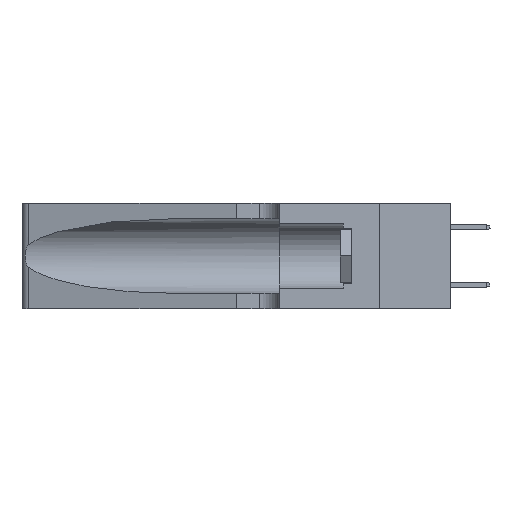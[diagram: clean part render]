
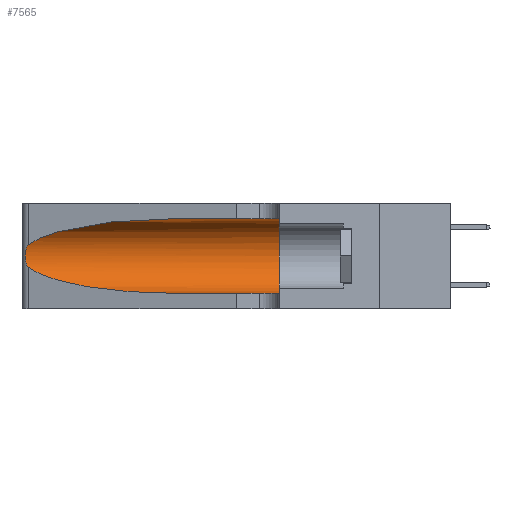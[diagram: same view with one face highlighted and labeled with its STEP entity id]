
A CAD part, left-side view. The second image highlights one B-rep face of the part: STEP entity #7565.
In plain terms, the highlighted cylindrical face has radius 3.308 mm (diameter 6.617 mm), a partial arc.
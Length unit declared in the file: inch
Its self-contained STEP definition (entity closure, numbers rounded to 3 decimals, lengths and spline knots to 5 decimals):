
#405 =( BOUNDED_CURVE ( )  B_SPLINE_CURVE ( 3, ( #37373, #41398, #25965, #8389 ),
 .UNSPECIFIED., .F., .T. ) 
 B_SPLINE_CURVE_WITH_KNOTS ( ( 4, 4 ),
 ( 1.5708, 2.84003 ),
 .UNSPECIFIED. ) 
 CURVE ( )  GEOMETRIC_REPRESENTATION_ITEM ( )  RATIONAL_B_SPLINE_CURVE ( ( 1., 0.87, 0.87, 1. ) ) 
 REPRESENTATION_ITEM ( '' )  );
#456 = CARTESIAN_POINT ( 'NONE',  ( 0.1305, 1.61858, 0.185 ) ) ;
#863 = DIRECTION ( 'NONE',  ( 0., -1., 0. ) ) ;
#1605 = CARTESIAN_POINT ( 'NONE',  ( 0.1305, 0.72297, 0.05475 ) ) ;
#2147 = CIRCLE ( 'NONE', #30199, 0.13025 ) ;
#2253 = CARTESIAN_POINT ( 'NONE',  ( 0.1305, 0.72297, 0.31525 ) ) ;
#2636 = EDGE_CURVE ( 'NONE', #8098, #27997, #2147, .T. ) ;
#3401 = CARTESIAN_POINT ( 'NONE',  ( 0.25789, 1.23486, 0.15765 ) ) ;
#3547 = EDGE_CURVE ( 'NONE', #12469, #27997, #24114, .T. ) ;
#4319 = EDGE_CURVE ( 'NONE', #40891, #12469, #14695, .T. ) ;
#4359 = CARTESIAN_POINT ( 'NONE',  ( 0.1305, 0.72297, 0.05475 ) ) ;
#4666 = LINE ( 'NONE', #18944, #4893 ) ;
#4893 = VECTOR ( 'NONE', #863, 39.37008 ) ;
#6642 = CARTESIAN_POINT ( 'NONE',  ( 0.1305, 0.35, 0.185 ) ) ;
#6947 = CARTESIAN_POINT ( 'NONE',  ( 0.26017, 1.23833, 0.17102 ) ) ;
#7431 = CARTESIAN_POINT ( 'NONE',  ( 0.26018, 1.23835, 0.19895 ) ) ;
#7565 = ADVANCED_FACE ( 'NONE', ( #22329 ), #33008, .F. ) ;
#8098 = VERTEX_POINT ( 'NONE', #11119 ) ;
#8389 = CARTESIAN_POINT ( 'NONE',  ( 0.25487, 1.22718, 0.22369 ) ) ;
#8571 = EDGE_LOOP ( 'NONE', ( #9879, #26465, #32762, #14339, #31455, #34783 ) ) ;
#9879 = ORIENTED_EDGE ( 'NONE', *, *, #27897, .T. ) ;
#10057 = VERTEX_POINT ( 'NONE', #12713 ) ;
#11119 = CARTESIAN_POINT ( 'NONE',  ( 0.1305, 0.35, 0.31525 ) ) ;
#12469 = VERTEX_POINT ( 'NONE', #4359 ) ;
#12713 = CARTESIAN_POINT ( 'NONE',  ( 0.25487, 1.22718, 0.22369 ) ) ;
#13401 = CARTESIAN_POINT ( 'NONE',  ( 0.25487, 1.22718, 0.22369 ) ) ;
#14079 = EDGE_CURVE ( 'NONE', #10057, #40891, #15015, .T. ) ;
#14339 = ORIENTED_EDGE ( 'NONE', *, *, #3547, .T. ) ;
#14544 = CARTESIAN_POINT ( 'NONE',  ( 0.25555, 1.22993, 0.14849 ) ) ;
#14695 =( BOUNDED_CURVE ( )  B_SPLINE_CURVE ( 3, ( #37728, #19687, #34153, #1605 ),
 .UNSPECIFIED., .F., .F. ) 
 B_SPLINE_CURVE_WITH_KNOTS ( ( 4, 4 ),
 ( 3.44316, 4.71239 ),
 .UNSPECIFIED. ) 
 CURVE ( )  GEOMETRIC_REPRESENTATION_ITEM ( )  RATIONAL_B_SPLINE_CURVE ( ( 1., 0.87, 0.87, 1. ) ) 
 REPRESENTATION_ITEM ( '' )  );
#15015 = B_SPLINE_CURVE_WITH_KNOTS ( 'NONE', 3,
 ( #13401, #27882, #42360, #38810, #20784, #7431, #21231, #43064, #6947, #24557, #3401, #36400, #14544, #18153 ),
 .UNSPECIFIED., .F., .F.,
 ( 4, 2, 2, 2, 2, 2, 4 ),
 ( 0., 0.00027, 0.00053, 0.00107, 0.0016, 0.00187, 0.00214 ),
 .UNSPECIFIED. ) ;
#16765 = CARTESIAN_POINT ( 'NONE',  ( 0.1305, 1.61858, 0.05475 ) ) ;
#18153 = CARTESIAN_POINT ( 'NONE',  ( 0.25487, 1.22718, 0.14631 ) ) ;
#18765 = DIRECTION ( 'NONE',  ( 0., 0., -1. ) ) ;
#18944 = CARTESIAN_POINT ( 'NONE',  ( 0.1305, 1.61858, 0.31525 ) ) ;
#19687 = CARTESIAN_POINT ( 'NONE',  ( 0.2373, 1.15595, 0.08982 ) ) ;
#20686 = DIRECTION ( 'NONE',  ( 0., 1., 0. ) ) ;
#20784 = CARTESIAN_POINT ( 'NONE',  ( 0.25854, 1.2359, 0.20912 ) ) ;
#21231 = CARTESIAN_POINT ( 'NONE',  ( 0.26075, 1.23896, 0.19203 ) ) ;
#22233 = AXIS2_PLACEMENT_3D ( 'NONE', #456, #40574, #18765 ) ;
#22329 = FACE_OUTER_BOUND ( 'NONE', #8571, .T. ) ;
#24114 = LINE ( 'NONE', #16765, #38634 ) ;
#24557 = CARTESIAN_POINT ( 'NONE',  ( 0.25856, 1.23593, 0.16098 ) ) ;
#25965 = CARTESIAN_POINT ( 'NONE',  ( 0.2373, 1.15595, 0.28018 ) ) ;
#26465 = ORIENTED_EDGE ( 'NONE', *, *, #14079, .T. ) ;
#27882 = CARTESIAN_POINT ( 'NONE',  ( 0.25555, 1.22994, 0.2215 ) ) ;
#27897 = EDGE_CURVE ( 'NONE', #35813, #10057, #405, .T. ) ;
#27997 = VERTEX_POINT ( 'NONE', #44036 ) ;
#30199 = AXIS2_PLACEMENT_3D ( 'NONE', #6642, #20686, #42038 ) ;
#31455 = ORIENTED_EDGE ( 'NONE', *, *, #2636, .F. ) ;
#32762 = ORIENTED_EDGE ( 'NONE', *, *, #4319, .T. ) ;
#33008 = CYLINDRICAL_SURFACE ( 'NONE', #22233, 0.13025 ) ;
#34153 = CARTESIAN_POINT ( 'NONE',  ( 0.18966, 0.96281, 0.05475 ) ) ;
#34783 = ORIENTED_EDGE ( 'NONE', *, *, #37734, .F. ) ;
#35813 = VERTEX_POINT ( 'NONE', #2253 ) ;
#36400 = CARTESIAN_POINT ( 'NONE',  ( 0.25639, 1.23186, 0.15144 ) ) ;
#37373 = CARTESIAN_POINT ( 'NONE',  ( 0.1305, 0.72297, 0.31525 ) ) ;
#37728 = CARTESIAN_POINT ( 'NONE',  ( 0.25487, 1.22718, 0.14631 ) ) ;
#37734 = EDGE_CURVE ( 'NONE', #35813, #8098, #4666, .T. ) ;
#38122 = DIRECTION ( 'NONE',  ( 0., -1., 0. ) ) ;
#38634 = VECTOR ( 'NONE', #38122, 39.37008 ) ;
#38810 = CARTESIAN_POINT ( 'NONE',  ( 0.25787, 1.23484, 0.2124 ) ) ;
#40574 = DIRECTION ( 'NONE',  ( 0., -1., 0. ) ) ;
#40891 = VERTEX_POINT ( 'NONE', #46855 ) ;
#41398 = CARTESIAN_POINT ( 'NONE',  ( 0.18966, 0.96281, 0.31525 ) ) ;
#42038 = DIRECTION ( 'NONE',  ( 0., 0., 1. ) ) ;
#42360 = CARTESIAN_POINT ( 'NONE',  ( 0.25639, 1.23184, 0.21858 ) ) ;
#43064 = CARTESIAN_POINT ( 'NONE',  ( 0.26075, 1.23896, 0.178 ) ) ;
#44036 = CARTESIAN_POINT ( 'NONE',  ( 0.1305, 0.35, 0.05475 ) ) ;
#46855 = CARTESIAN_POINT ( 'NONE',  ( 0.25487, 1.22718, 0.14631 ) ) ;
